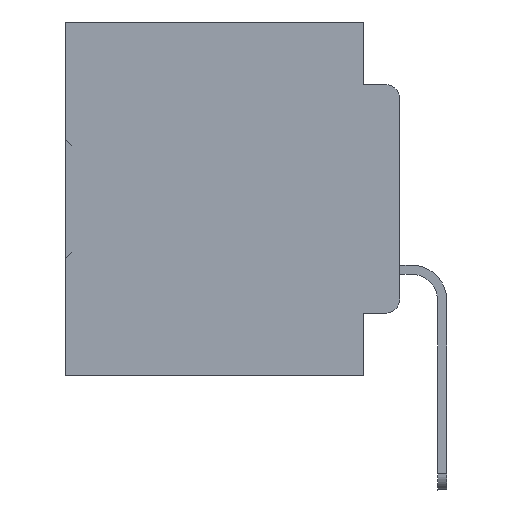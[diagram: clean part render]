
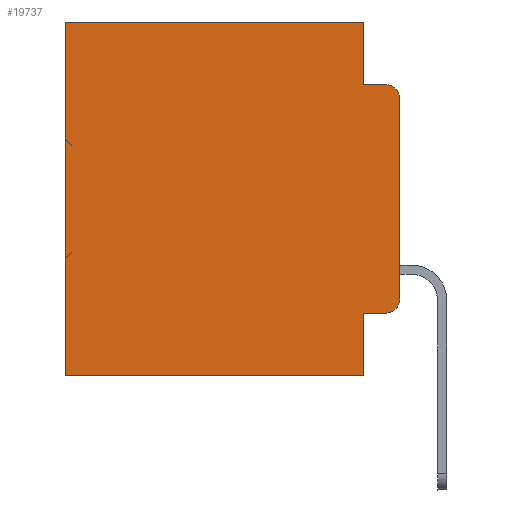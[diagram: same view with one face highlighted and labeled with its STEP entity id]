
A CAD part, left-side view. The second image highlights one B-rep face of the part: STEP entity #19737.
In plain terms, the highlighted planar face has unit normal (-1, 0, 0).
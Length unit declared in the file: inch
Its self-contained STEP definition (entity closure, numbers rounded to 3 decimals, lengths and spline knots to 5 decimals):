
#439 = CARTESIAN_POINT ( 'NONE',  ( 0.298, 0.02, -0.3915 ) ) ;
#1730 = VERTEX_POINT ( 'NONE', #12221 ) ;
#1815 = LINE ( 'NONE', #35079, #31526 ) ;
#2356 = EDGE_CURVE ( 'NONE', #33320, #21650, #30485, .T. ) ;
#2408 = FACE_OUTER_BOUND ( 'NONE', #17266, .T. ) ;
#2761 = CARTESIAN_POINT ( 'NONE',  ( 0.298, 0.02, -0.4115 ) ) ;
#3972 = ORIENTED_EDGE ( 'NONE', *, *, #31505, .T. ) ;
#5243 = VECTOR ( 'NONE', #34492, 39.37008 ) ;
#5413 = DIRECTION ( 'NONE',  ( 0., -1., 0. ) ) ;
#5443 = EDGE_CURVE ( 'NONE', #9758, #13025, #32532, .T. ) ;
#5815 = CIRCLE ( 'NONE', #26909, 0.02 ) ;
#5880 = VECTOR ( 'NONE', #29145, 39.37008 ) ;
#6153 = VERTEX_POINT ( 'NONE', #17157 ) ;
#6644 = EDGE_CURVE ( 'NONE', #9758, #7672, #6685, .T. ) ;
#6685 = LINE ( 'NONE', #30095, #35790 ) ;
#6723 = CARTESIAN_POINT ( 'NONE',  ( 0.298, 0.051, -0.5 ) ) ;
#6861 = DIRECTION ( 'NONE',  ( 0., 0., -1. ) ) ;
#6879 = CARTESIAN_POINT ( 'NONE',  ( 0.298, 0.051, 0. ) ) ;
#7672 = VERTEX_POINT ( 'NONE', #36197 ) ;
#7798 = CARTESIAN_POINT ( 'NONE',  ( 0.298, 0.02, -0.0885 ) ) ;
#8820 = CARTESIAN_POINT ( 'NONE',  ( 0.298, 0.051, -0.0885 ) ) ;
#9512 = AXIS2_PLACEMENT_3D ( 'NONE', #439, #13715, #12132 ) ;
#9536 = LINE ( 'NONE', #6879, #5880 ) ;
#9758 = VERTEX_POINT ( 'NONE', #11993 ) ;
#9852 = CARTESIAN_POINT ( 'NONE',  ( 0.298, 0.051, -0.0885 ) ) ;
#10425 = ORIENTED_EDGE ( 'NONE', *, *, #2356, .F. ) ;
#11418 = CARTESIAN_POINT ( 'NONE',  ( 0.298, 0.473, -0.5 ) ) ;
#11464 = VERTEX_POINT ( 'NONE', #2761 ) ;
#11894 = CIRCLE ( 'NONE', #9512, 0.02 ) ;
#11993 = CARTESIAN_POINT ( 'NONE',  ( 0.298, 0.051, 0. ) ) ;
#12018 = LINE ( 'NONE', #8820, #19503 ) ;
#12132 = DIRECTION ( 'NONE',  ( 0., 0., -1. ) ) ;
#12221 = CARTESIAN_POINT ( 'NONE',  ( 0.298, 0.051, -0.4115 ) ) ;
#13025 = VERTEX_POINT ( 'NONE', #9852 ) ;
#13228 = ORIENTED_EDGE ( 'NONE', *, *, #6644, .T. ) ;
#13715 = DIRECTION ( 'NONE',  ( -1., 0., 0. ) ) ;
#13718 = ORIENTED_EDGE ( 'NONE', *, *, #34225, .F. ) ;
#13914 = PLANE ( 'NONE',  #14861 ) ;
#14587 = ORIENTED_EDGE ( 'NONE', *, *, #5443, .F. ) ;
#14861 = AXIS2_PLACEMENT_3D ( 'NONE', #26166, #34662, #23342 ) ;
#15341 = ORIENTED_EDGE ( 'NONE', *, *, #27405, .T. ) ;
#15870 = EDGE_CURVE ( 'NONE', #13025, #19342, #12018, .T. ) ;
#16494 = CARTESIAN_POINT ( 'NONE',  ( 0.298, 0., -0.5 ) ) ;
#17157 = CARTESIAN_POINT ( 'NONE',  ( 0.298, 0., -0.1085 ) ) ;
#17266 = EDGE_LOOP ( 'NONE', ( #13718, #28734, #25354, #14587, #13228, #3972, #10425, #25878, #15341, #22049 ) ) ;
#17547 = CARTESIAN_POINT ( 'NONE',  ( 0.298, 0.02, -0.1085 ) ) ;
#18045 = DIRECTION ( 'NONE',  ( 0., -1., 0. ) ) ;
#19342 = VERTEX_POINT ( 'NONE', #7798 ) ;
#19503 = VECTOR ( 'NONE', #18045, 39.37008 ) ;
#19737 = ADVANCED_FACE ( 'NONE', ( #2408 ), #13914, .F. ) ;
#19781 = CARTESIAN_POINT ( 'NONE',  ( 0.298, 0.473, 0. ) ) ;
#20331 = EDGE_CURVE ( 'NONE', #1730, #33320, #9536, .T. ) ;
#21338 = VECTOR ( 'NONE', #5413, 39.37008 ) ;
#21650 = VERTEX_POINT ( 'NONE', #11418 ) ;
#22049 = ORIENTED_EDGE ( 'NONE', *, *, #31966, .T. ) ;
#23342 = DIRECTION ( 'NONE',  ( 0., 0., -1. ) ) ;
#23348 = LINE ( 'NONE', #19781, #5243 ) ;
#25354 = ORIENTED_EDGE ( 'NONE', *, *, #15870, .F. ) ;
#25878 = ORIENTED_EDGE ( 'NONE', *, *, #20331, .F. ) ;
#26166 = CARTESIAN_POINT ( 'NONE',  ( 0.298, 0., 0. ) ) ;
#26744 = CARTESIAN_POINT ( 'NONE',  ( 0.298, 0., -0.3915 ) ) ;
#26909 = AXIS2_PLACEMENT_3D ( 'NONE', #17547, #36170, #32468 ) ;
#27246 = DIRECTION ( 'NONE',  ( 0., 1., 0. ) ) ;
#27405 = EDGE_CURVE ( 'NONE', #1730, #11464, #28434, .T. ) ;
#28434 = LINE ( 'NONE', #31270, #21338 ) ;
#28734 = ORIENTED_EDGE ( 'NONE', *, *, #29958, .T. ) ;
#29145 = DIRECTION ( 'NONE',  ( 0., 0., -1. ) ) ;
#29699 = CARTESIAN_POINT ( 'NONE',  ( 0.298, 0.051, 0. ) ) ;
#29958 = EDGE_CURVE ( 'NONE', #6153, #19342, #5815, .T. ) ;
#30095 = CARTESIAN_POINT ( 'NONE',  ( 0.298, 0., 0. ) ) ;
#30485 = LINE ( 'NONE', #16494, #33663 ) ;
#31270 = CARTESIAN_POINT ( 'NONE',  ( 0.298, 0.051, -0.4115 ) ) ;
#31505 = EDGE_CURVE ( 'NONE', #7672, #21650, #23348, .T. ) ;
#31526 = VECTOR ( 'NONE', #32258, 39.37008 ) ;
#31966 = EDGE_CURVE ( 'NONE', #11464, #37103, #11894, .T. ) ;
#32073 = VECTOR ( 'NONE', #6861, 39.37008 ) ;
#32258 = DIRECTION ( 'NONE',  ( 0., 0., -1. ) ) ;
#32468 = DIRECTION ( 'NONE',  ( 0., 0., -1. ) ) ;
#32532 = LINE ( 'NONE', #29699, #32073 ) ;
#33308 = DIRECTION ( 'NONE',  ( 0., 1., 0. ) ) ;
#33320 = VERTEX_POINT ( 'NONE', #6723 ) ;
#33663 = VECTOR ( 'NONE', #33308, 39.37008 ) ;
#34225 = EDGE_CURVE ( 'NONE', #6153, #37103, #1815, .T. ) ;
#34492 = DIRECTION ( 'NONE',  ( 0., 0., -1. ) ) ;
#34662 = DIRECTION ( 'NONE',  ( 1., 0., 0. ) ) ;
#35079 = CARTESIAN_POINT ( 'NONE',  ( 0.298, 0., 0. ) ) ;
#35790 = VECTOR ( 'NONE', #27246, 39.37008 ) ;
#36170 = DIRECTION ( 'NONE',  ( -1., 0., 0. ) ) ;
#36197 = CARTESIAN_POINT ( 'NONE',  ( 0.298, 0.473, 0. ) ) ;
#37103 = VERTEX_POINT ( 'NONE', #26744 ) ;
